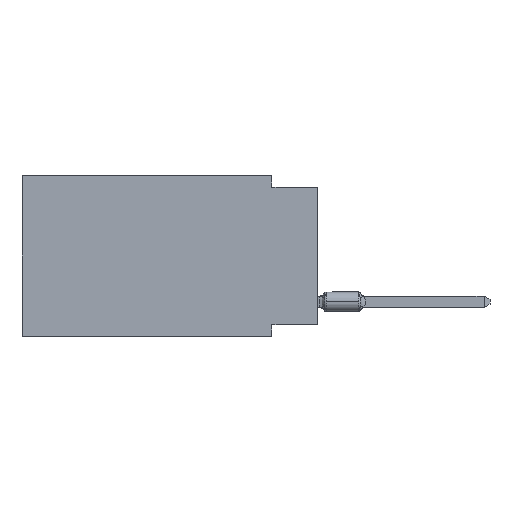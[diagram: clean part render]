
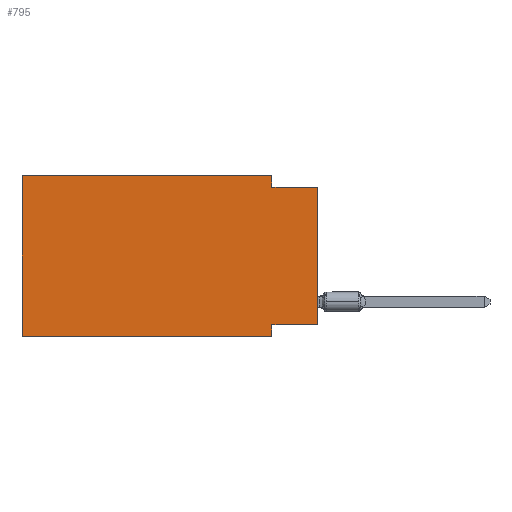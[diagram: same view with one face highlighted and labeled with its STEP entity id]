
A CAD part, left-side view. The second image highlights one B-rep face of the part: STEP entity #795.
In plain terms, the highlighted planar face has unit normal (-1, 0, 0).
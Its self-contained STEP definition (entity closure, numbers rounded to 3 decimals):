
#115 = DIRECTION ( 'NONE',  ( 0., -1., 0. ) ) ;
#172 = CARTESIAN_POINT ( 'NONE',  ( 0., 16.383, 0. ) ) ;
#521 = VERTEX_POINT ( 'NONE', #14606 ) ;
#774 = VECTOR ( 'NONE', #115, 1000. ) ;
#795 = ADVANCED_FACE ( 'NONE', ( #9510 ), #14291, .F. ) ;
#1116 = EDGE_CURVE ( 'NONE', #9080, #1369, #10258, .T. ) ;
#1268 = DIRECTION ( 'NONE',  ( 0., 1., 0. ) ) ;
#1269 = VERTEX_POINT ( 'NONE', #3944 ) ;
#1369 = VERTEX_POINT ( 'NONE', #7524 ) ;
#1616 = DIRECTION ( 'NONE',  ( 0., 0., -1. ) ) ;
#1768 = VECTOR ( 'NONE', #3219, 1000. ) ;
#1825 = EDGE_LOOP ( 'NONE', ( #8147, #8403, #8483, #9032, #6416, #2548, #2004, #14970 ) ) ;
#2004 = ORIENTED_EDGE ( 'NONE', *, *, #11786, .F. ) ;
#2548 = ORIENTED_EDGE ( 'NONE', *, *, #4839, .T. ) ;
#2817 = EDGE_CURVE ( 'NONE', #521, #11184, #3997, .T. ) ;
#3219 = DIRECTION ( 'NONE',  ( 0., -1., 0. ) ) ;
#3944 = CARTESIAN_POINT ( 'NONE',  ( 0., 2.54, 0. ) ) ;
#3997 = LINE ( 'NONE', #8645, #6172 ) ;
#4185 = CARTESIAN_POINT ( 'NONE',  ( 0., 0., -8.255 ) ) ;
#4442 = LINE ( 'NONE', #13186, #1768 ) ;
#4839 = EDGE_CURVE ( 'NONE', #521, #9524, #6328, .T. ) ;
#5699 = EDGE_CURVE ( 'NONE', #11097, #1369, #4442, .T. ) ;
#5719 = DIRECTION ( 'NONE',  ( 0., 0., 1. ) ) ;
#5759 = VECTOR ( 'NONE', #5719, 1000. ) ;
#5776 = CARTESIAN_POINT ( 'NONE',  ( 0., 2.54, -8.89 ) ) ;
#6172 = VECTOR ( 'NONE', #7662, 1000. ) ;
#6328 = LINE ( 'NONE', #12165, #9305 ) ;
#6416 = ORIENTED_EDGE ( 'NONE', *, *, #2817, .F. ) ;
#6840 = VECTOR ( 'NONE', #12653, 1000. ) ;
#7042 = LINE ( 'NONE', #11670, #9021 ) ;
#7248 = DIRECTION ( 'NONE',  ( 1., 0., 0. ) ) ;
#7292 = LINE ( 'NONE', #7590, #13682 ) ;
#7524 = CARTESIAN_POINT ( 'NONE',  ( 0., 0., -0.635 ) ) ;
#7540 = CARTESIAN_POINT ( 'NONE',  ( 0., 16.383, 0. ) ) ;
#7590 = CARTESIAN_POINT ( 'NONE',  ( 0., 2.54, 0. ) ) ;
#7649 = EDGE_CURVE ( 'NONE', #1269, #11097, #7292, .T. ) ;
#7662 = DIRECTION ( 'NONE',  ( 0., 0., 1. ) ) ;
#7688 = AXIS2_PLACEMENT_3D ( 'NONE', #172, #7248, #1616 ) ;
#8147 = ORIENTED_EDGE ( 'NONE', *, *, #1116, .T. ) ;
#8403 = ORIENTED_EDGE ( 'NONE', *, *, #5699, .F. ) ;
#8483 = ORIENTED_EDGE ( 'NONE', *, *, #7649, .F. ) ;
#8645 = CARTESIAN_POINT ( 'NONE',  ( 0., 16.383, 0. ) ) ;
#9021 = VECTOR ( 'NONE', #1268, 1000. ) ;
#9032 = ORIENTED_EDGE ( 'NONE', *, *, #12207, .F. ) ;
#9080 = VERTEX_POINT ( 'NONE', #4185 ) ;
#9106 = LINE ( 'NONE', #5776, #6840 ) ;
#9305 = VECTOR ( 'NONE', #14739, 1000. ) ;
#9510 = FACE_OUTER_BOUND ( 'NONE', #1825, .T. ) ;
#9524 = VERTEX_POINT ( 'NONE', #10371 ) ;
#9825 = VERTEX_POINT ( 'NONE', #12181 ) ;
#10258 = LINE ( 'NONE', #11403, #5759 ) ;
#10371 = CARTESIAN_POINT ( 'NONE',  ( 0., 2.54, -8.89 ) ) ;
#10527 = CARTESIAN_POINT ( 'NONE',  ( 0., 16.383, 0. ) ) ;
#11097 = VERTEX_POINT ( 'NONE', #13365 ) ;
#11184 = VERTEX_POINT ( 'NONE', #7540 ) ;
#11403 = CARTESIAN_POINT ( 'NONE',  ( 0., 0., 0. ) ) ;
#11668 = LINE ( 'NONE', #10527, #774 ) ;
#11670 = CARTESIAN_POINT ( 'NONE',  ( 0., 0., -8.255 ) ) ;
#11786 = EDGE_CURVE ( 'NONE', #9825, #9524, #9106, .T. ) ;
#12165 = CARTESIAN_POINT ( 'NONE',  ( 0., 16.383, -8.89 ) ) ;
#12181 = CARTESIAN_POINT ( 'NONE',  ( 0., 2.54, -8.255 ) ) ;
#12207 = EDGE_CURVE ( 'NONE', #11184, #1269, #11668, .T. ) ;
#12653 = DIRECTION ( 'NONE',  ( 0., 0., -1. ) ) ;
#13186 = CARTESIAN_POINT ( 'NONE',  ( 0., 0., -0.635 ) ) ;
#13190 = DIRECTION ( 'NONE',  ( 0., 0., -1. ) ) ;
#13365 = CARTESIAN_POINT ( 'NONE',  ( 0., 2.54, -0.635 ) ) ;
#13420 = EDGE_CURVE ( 'NONE', #9080, #9825, #7042, .T. ) ;
#13682 = VECTOR ( 'NONE', #13190, 1000. ) ;
#14291 = PLANE ( 'NONE',  #7688 ) ;
#14606 = CARTESIAN_POINT ( 'NONE',  ( 0., 16.383, -8.89 ) ) ;
#14739 = DIRECTION ( 'NONE',  ( 0., -1., 0. ) ) ;
#14970 = ORIENTED_EDGE ( 'NONE', *, *, #13420, .F. ) ;
